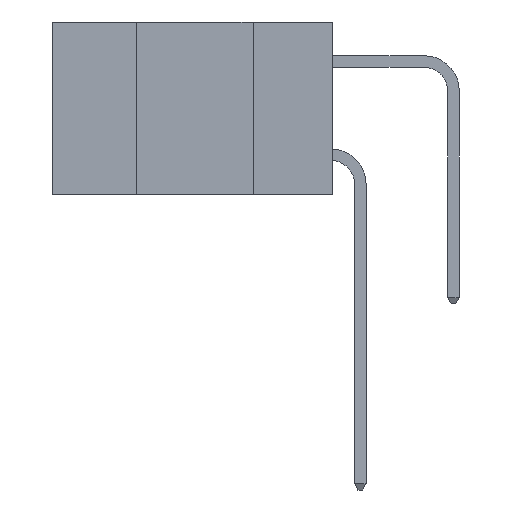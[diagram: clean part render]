
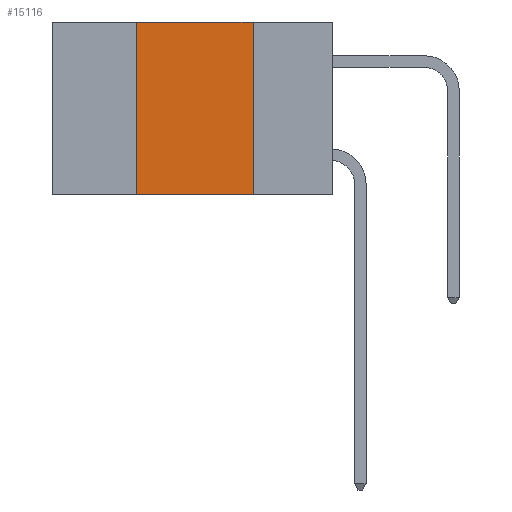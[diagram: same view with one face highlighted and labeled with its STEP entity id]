
A CAD part, left-side view. The second image highlights one B-rep face of the part: STEP entity #15116.
In plain terms, the highlighted planar face has unit normal (-1, 0, 0).
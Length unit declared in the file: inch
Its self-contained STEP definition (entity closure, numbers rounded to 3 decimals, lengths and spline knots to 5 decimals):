
#1265 = CARTESIAN_POINT ( 'NONE',  ( 0., 0.42, 0. ) ) ;
#2416 = DIRECTION ( 'NONE',  ( 0., 0., -1. ) ) ;
#3116 = VECTOR ( 'NONE', #18684, 39.37008 ) ;
#4070 = VERTEX_POINT ( 'NONE', #9583 ) ;
#4210 = EDGE_CURVE ( 'NONE', #17291, #13710, #5570, .T. ) ;
#5570 = LINE ( 'NONE', #6143, #20984 ) ;
#5936 = VECTOR ( 'NONE', #9747, 39.37008 ) ;
#5945 = FACE_OUTER_BOUND ( 'NONE', #8863, .T. ) ;
#6115 = CARTESIAN_POINT ( 'NONE',  ( 0., 0.17, -0.37 ) ) ;
#6143 = CARTESIAN_POINT ( 'NONE',  ( 0., 0.6, 0. ) ) ;
#6289 = DIRECTION ( 'NONE',  ( 0., 0., -1. ) ) ;
#8110 = ORIENTED_EDGE ( 'NONE', *, *, #4210, .F. ) ;
#8374 = ORIENTED_EDGE ( 'NONE', *, *, #20798, .F. ) ;
#8863 = EDGE_LOOP ( 'NONE', ( #13329, #8110, #8374, #9550 ) ) ;
#9550 = ORIENTED_EDGE ( 'NONE', *, *, #25798, .T. ) ;
#9583 = CARTESIAN_POINT ( 'NONE',  ( 0., 0.42, -0.37 ) ) ;
#9747 = DIRECTION ( 'NONE',  ( 0., 0., 1. ) ) ;
#10315 = CARTESIAN_POINT ( 'NONE',  ( 0., 0.6, -0.37 ) ) ;
#11181 = CARTESIAN_POINT ( 'NONE',  ( 0., 0.17, 0. ) ) ;
#12382 = VECTOR ( 'NONE', #2416, 39.37008 ) ;
#12508 = AXIS2_PLACEMENT_3D ( 'NONE', #24971, #18857, #6289 ) ;
#12984 = CARTESIAN_POINT ( 'NONE',  ( 0., 0.17, -0.37 ) ) ;
#13009 = LINE ( 'NONE', #12984, #12382 ) ;
#13329 = ORIENTED_EDGE ( 'NONE', *, *, #18138, .F. ) ;
#13710 = VERTEX_POINT ( 'NONE', #11181 ) ;
#14373 = LINE ( 'NONE', #10315, #3116 ) ;
#14622 = DIRECTION ( 'NONE',  ( 0., -1., 0. ) ) ;
#15116 = ADVANCED_FACE ( 'NONE', ( #5945 ), #16786, .F. ) ;
#16786 = PLANE ( 'NONE',  #12508 ) ;
#17118 = LINE ( 'NONE', #26449, #5936 ) ;
#17291 = VERTEX_POINT ( 'NONE', #1265 ) ;
#18138 = EDGE_CURVE ( 'NONE', #13710, #18596, #13009, .T. ) ;
#18596 = VERTEX_POINT ( 'NONE', #6115 ) ;
#18684 = DIRECTION ( 'NONE',  ( 0., -1., 0. ) ) ;
#18857 = DIRECTION ( 'NONE',  ( 1., 0., 0. ) ) ;
#20798 = EDGE_CURVE ( 'NONE', #4070, #17291, #17118, .T. ) ;
#20984 = VECTOR ( 'NONE', #14622, 39.37008 ) ;
#24971 = CARTESIAN_POINT ( 'NONE',  ( 0., 0.6, 0. ) ) ;
#25798 = EDGE_CURVE ( 'NONE', #4070, #18596, #14373, .T. ) ;
#26449 = CARTESIAN_POINT ( 'NONE',  ( 0., 0.42, -0.37 ) ) ;
